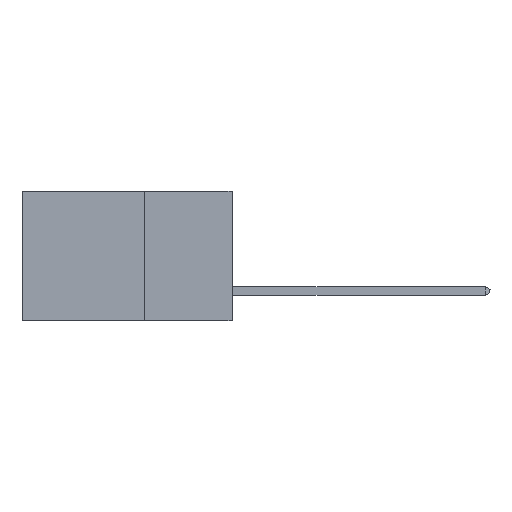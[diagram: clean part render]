
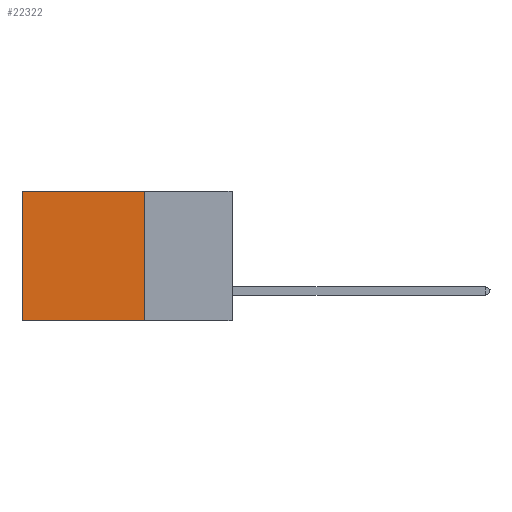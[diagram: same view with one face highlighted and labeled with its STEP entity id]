
A CAD part, left-side view. The second image highlights one B-rep face of the part: STEP entity #22322.
In plain terms, the highlighted planar face has unit normal (-1, 0, 0).
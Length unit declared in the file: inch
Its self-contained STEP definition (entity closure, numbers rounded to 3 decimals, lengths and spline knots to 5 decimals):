
#72 = DIRECTION ( 'NONE',  ( 0., 1., 0. ) ) ;
#295 = CARTESIAN_POINT ( 'NONE',  ( 0.2875, 0.25, 0. ) ) ;
#1071 = ORIENTED_EDGE ( 'NONE', *, *, #34760, .T. ) ;
#1409 = ORIENTED_EDGE ( 'NONE', *, *, #36357, .T. ) ;
#2394 = CARTESIAN_POINT ( 'NONE',  ( 0.2875, 0.6, 0. ) ) ;
#2860 = EDGE_CURVE ( 'NONE', #39661, #12881, #7345, .T. ) ;
#3270 = PLANE ( 'NONE',  #10491 ) ;
#5556 = CARTESIAN_POINT ( 'NONE',  ( 0.2875, 0.25, -0.37 ) ) ;
#6205 = CARTESIAN_POINT ( 'NONE',  ( 0.2875, 0.6, 0. ) ) ;
#7345 = LINE ( 'NONE', #17693, #26363 ) ;
#9461 = DIRECTION ( 'NONE',  ( 1., 0., 0. ) ) ;
#9516 = FACE_OUTER_BOUND ( 'NONE', #41342, .T. ) ;
#9981 = VECTOR ( 'NONE', #17352, 39.37008 ) ;
#10491 = AXIS2_PLACEMENT_3D ( 'NONE', #28826, #9461, #28959 ) ;
#11602 = ORIENTED_EDGE ( 'NONE', *, *, #2860, .F. ) ;
#12881 = VERTEX_POINT ( 'NONE', #19228 ) ;
#13333 = VERTEX_POINT ( 'NONE', #22128 ) ;
#14545 = ORIENTED_EDGE ( 'NONE', *, *, #36933, .F. ) ;
#17352 = DIRECTION ( 'NONE',  ( 0., 0., -1. ) ) ;
#17693 = CARTESIAN_POINT ( 'NONE',  ( 0.2875, 0.25, -0.37 ) ) ;
#18915 = VECTOR ( 'NONE', #19282, 39.37008 ) ;
#19228 = CARTESIAN_POINT ( 'NONE',  ( 0.2875, 0.6, -0.37 ) ) ;
#19282 = DIRECTION ( 'NONE',  ( 0., 1., 0. ) ) ;
#22128 = CARTESIAN_POINT ( 'NONE',  ( 0.2875, 0.25, 0. ) ) ;
#22322 = ADVANCED_FACE ( 'NONE', ( #9516 ), #3270, .F. ) ;
#23968 = VECTOR ( 'NONE', #27822, 39.37008 ) ;
#24923 = LINE ( 'NONE', #295, #18915 ) ;
#26363 = VECTOR ( 'NONE', #72, 39.37008 ) ;
#27822 = DIRECTION ( 'NONE',  ( 0., 0., -1. ) ) ;
#28595 = LINE ( 'NONE', #36524, #9981 ) ;
#28826 = CARTESIAN_POINT ( 'NONE',  ( 0.2875, 0.25, 0. ) ) ;
#28959 = DIRECTION ( 'NONE',  ( 0., 0., -1. ) ) ;
#34760 = EDGE_CURVE ( 'NONE', #39579, #12881, #38503, .T. ) ;
#36357 = EDGE_CURVE ( 'NONE', #13333, #39579, #24923, .T. ) ;
#36524 = CARTESIAN_POINT ( 'NONE',  ( 0.2875, 0.25, 0. ) ) ;
#36933 = EDGE_CURVE ( 'NONE', #13333, #39661, #28595, .T. ) ;
#38503 = LINE ( 'NONE', #2394, #23968 ) ;
#39579 = VERTEX_POINT ( 'NONE', #6205 ) ;
#39661 = VERTEX_POINT ( 'NONE', #5556 ) ;
#41342 = EDGE_LOOP ( 'NONE', ( #1071, #11602, #14545, #1409 ) ) ;
